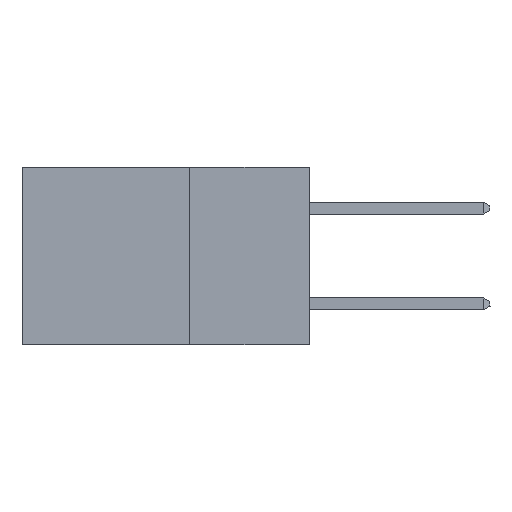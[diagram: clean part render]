
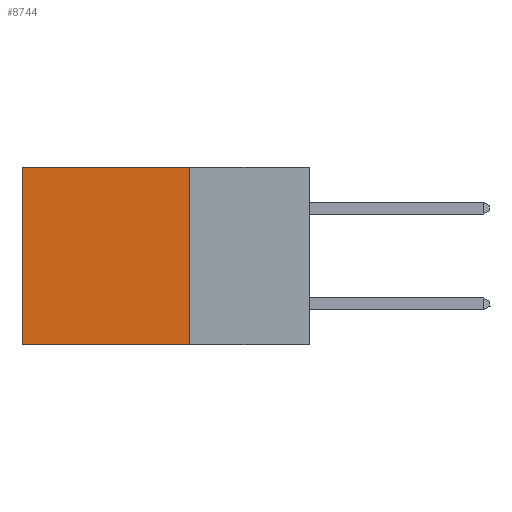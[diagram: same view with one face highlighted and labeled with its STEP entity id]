
A CAD part, left-side view. The second image highlights one B-rep face of the part: STEP entity #8744.
In plain terms, the highlighted planar face has unit normal (-1, 0, 0).
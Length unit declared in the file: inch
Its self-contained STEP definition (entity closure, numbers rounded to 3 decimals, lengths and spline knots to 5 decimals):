
#90 = EDGE_LOOP ( 'NONE', ( #18990, #2282, #6560, #5357 ) ) ;
#314 = CARTESIAN_POINT ( 'NONE',  ( 0.2875, 0.6, 0. ) ) ;
#2282 = ORIENTED_EDGE ( 'NONE', *, *, #25188, .F. ) ;
#2633 = PLANE ( 'NONE',  #12764 ) ;
#3038 = VECTOR ( 'NONE', #5940, 39.37008 ) ;
#3210 = EDGE_CURVE ( 'NONE', #19466, #15160, #20826, .T. ) ;
#3678 = CARTESIAN_POINT ( 'NONE',  ( 0.2875, 0.25, -0.37 ) ) ;
#4808 = CARTESIAN_POINT ( 'NONE',  ( 0.2875, 0.25, 0. ) ) ;
#5357 = ORIENTED_EDGE ( 'NONE', *, *, #21558, .T. ) ;
#5494 = LINE ( 'NONE', #3678, #3038 ) ;
#5630 = EDGE_CURVE ( 'NONE', #27790, #17438, #25497, .T. ) ;
#5940 = DIRECTION ( 'NONE',  ( 0., 1., 0. ) ) ;
#6560 = ORIENTED_EDGE ( 'NONE', *, *, #5630, .F. ) ;
#7117 = DIRECTION ( 'NONE',  ( 0., 0., -1. ) ) ;
#8744 = ADVANCED_FACE ( 'NONE', ( #20018 ), #2633, .F. ) ;
#11574 = DIRECTION ( 'NONE',  ( 1., 0., 0. ) ) ;
#12764 = AXIS2_PLACEMENT_3D ( 'NONE', #4808, #11574, #15801 ) ;
#12869 = CARTESIAN_POINT ( 'NONE',  ( 0.2875, 0.25, -0.37 ) ) ;
#14514 = VECTOR ( 'NONE', #7117, 39.37008 ) ;
#15160 = VERTEX_POINT ( 'NONE', #26287 ) ;
#15700 = DIRECTION ( 'NONE',  ( 0., 0., -1. ) ) ;
#15801 = DIRECTION ( 'NONE',  ( 0., 0., -1. ) ) ;
#16644 = CARTESIAN_POINT ( 'NONE',  ( 0.2875, 0.25, 0. ) ) ;
#17438 = VERTEX_POINT ( 'NONE', #12869 ) ;
#18990 = ORIENTED_EDGE ( 'NONE', *, *, #3210, .T. ) ;
#19466 = VERTEX_POINT ( 'NONE', #27139 ) ;
#19494 = VECTOR ( 'NONE', #15700, 39.37008 ) ;
#20018 = FACE_OUTER_BOUND ( 'NONE', #90, .T. ) ;
#20826 = LINE ( 'NONE', #314, #14514 ) ;
#21558 = EDGE_CURVE ( 'NONE', #27790, #19466, #28950, .T. ) ;
#22955 = VECTOR ( 'NONE', #23377, 39.37008 ) ;
#23377 = DIRECTION ( 'NONE',  ( 0., 1., 0. ) ) ;
#25002 = CARTESIAN_POINT ( 'NONE',  ( 0.2875, 0.25, 0. ) ) ;
#25188 = EDGE_CURVE ( 'NONE', #17438, #15160, #5494, .T. ) ;
#25300 = CARTESIAN_POINT ( 'NONE',  ( 0.2875, 0.25, 0. ) ) ;
#25497 = LINE ( 'NONE', #25002, #19494 ) ;
#26287 = CARTESIAN_POINT ( 'NONE',  ( 0.2875, 0.6, -0.37 ) ) ;
#27139 = CARTESIAN_POINT ( 'NONE',  ( 0.2875, 0.6, 0. ) ) ;
#27790 = VERTEX_POINT ( 'NONE', #25300 ) ;
#28950 = LINE ( 'NONE', #16644, #22955 ) ;
